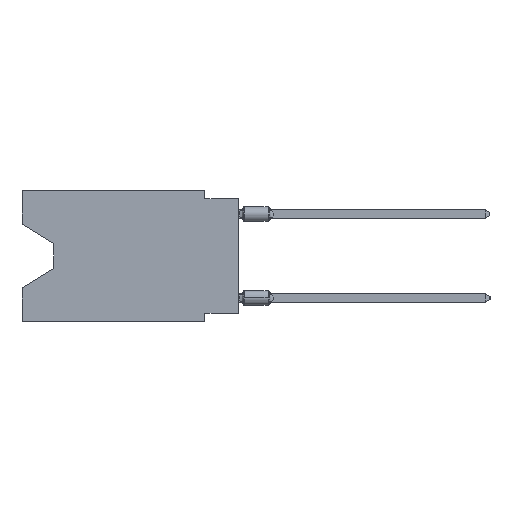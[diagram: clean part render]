
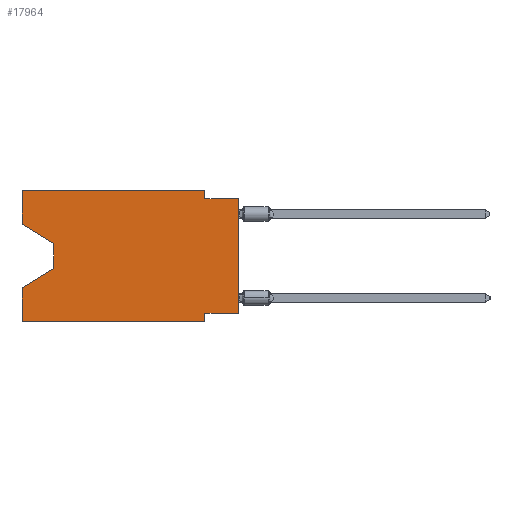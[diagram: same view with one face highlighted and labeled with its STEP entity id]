
A CAD part, left-side view. The second image highlights one B-rep face of the part: STEP entity #17964.
In plain terms, the highlighted planar face has unit normal (-1, 0, 0).
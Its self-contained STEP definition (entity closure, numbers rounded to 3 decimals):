
#2593 = LINE ( 'NONE', #3470, #9053 ) ;
#2955 = VERTEX_POINT ( 'NONE', #20344 ) ;
#3470 = CARTESIAN_POINT ( 'NONE',  ( 0., 0., -0.635 ) ) ;
#4074 = CARTESIAN_POINT ( 'NONE',  ( 0., 16.383, -2.546 ) ) ;
#4353 = LINE ( 'NONE', #4074, #47455 ) ;
#4602 = DIRECTION ( 'NONE',  ( 0., 1., 0. ) ) ;
#5202 = ORIENTED_EDGE ( 'NONE', *, *, #27880, .T. ) ;
#5480 = EDGE_CURVE ( 'NONE', #35340, #27642, #8712, .T. ) ;
#5612 = PLANE ( 'NONE',  #28601 ) ;
#5789 = DIRECTION ( 'NONE',  ( 0., -1., 0. ) ) ;
#5990 = ORIENTED_EDGE ( 'NONE', *, *, #41728, .F. ) ;
#7350 = EDGE_CURVE ( 'NONE', #36965, #53989, #55709, .T. ) ;
#8078 = VERTEX_POINT ( 'NONE', #9866 ) ;
#8114 = CARTESIAN_POINT ( 'NONE',  ( 0., 0., -9.271 ) ) ;
#8610 = EDGE_CURVE ( 'NONE', #47030, #40802, #19693, .T. ) ;
#8712 = LINE ( 'NONE', #17474, #56254 ) ;
#9053 = VECTOR ( 'NONE', #56425, 1000. ) ;
#9615 = VERTEX_POINT ( 'NONE', #36421 ) ;
#9800 = CARTESIAN_POINT ( 'NONE',  ( 0., 13.97, -4.013 ) ) ;
#9866 = CARTESIAN_POINT ( 'NONE',  ( 0., 13.97, -5.893 ) ) ;
#10075 = LINE ( 'NONE', #9800, #38184 ) ;
#10081 = CARTESIAN_POINT ( 'NONE',  ( 0., 2.54, 0. ) ) ;
#10205 = EDGE_CURVE ( 'NONE', #35075, #56431, #42723, .T. ) ;
#10977 = CARTESIAN_POINT ( 'NONE',  ( 0., 16.383, -2.546 ) ) ;
#11477 = CARTESIAN_POINT ( 'NONE',  ( 0., 16.383, -9.906 ) ) ;
#11584 = ORIENTED_EDGE ( 'NONE', *, *, #8610, .T. ) ;
#12892 = DIRECTION ( 'NONE',  ( 0., 0., 1. ) ) ;
#13068 = CARTESIAN_POINT ( 'NONE',  ( 0., 0., -0.635 ) ) ;
#13733 = VECTOR ( 'NONE', #12892, 1000. ) ;
#15483 = VECTOR ( 'NONE', #55414, 1000. ) ;
#16122 = CARTESIAN_POINT ( 'NONE',  ( 0., 16.383, 0. ) ) ;
#17239 = DIRECTION ( 'NONE',  ( 0., 0.855, -0.519 ) ) ;
#17474 = CARTESIAN_POINT ( 'NONE',  ( 0., 16.383, 0. ) ) ;
#17768 = DIRECTION ( 'NONE',  ( 0., 0., 1. ) ) ;
#17964 = ADVANCED_FACE ( 'NONE', ( #55345 ), #5612, .F. ) ;
#18504 = EDGE_CURVE ( 'NONE', #53989, #40802, #2593, .T. ) ;
#19154 = ORIENTED_EDGE ( 'NONE', *, *, #18504, .F. ) ;
#19693 = LINE ( 'NONE', #37544, #15483 ) ;
#20344 = CARTESIAN_POINT ( 'NONE',  ( 0., 13.97, -4.013 ) ) ;
#20824 = VECTOR ( 'NONE', #21401, 1000. ) ;
#21401 = DIRECTION ( 'NONE',  ( 0., -1., 0. ) ) ;
#22155 = EDGE_CURVE ( 'NONE', #47030, #34508, #52581, .T. ) ;
#23251 = ORIENTED_EDGE ( 'NONE', *, *, #31248, .T. ) ;
#23791 = DIRECTION ( 'NONE',  ( 0., 0., -1. ) ) ;
#25501 = LINE ( 'NONE', #11477, #20824 ) ;
#25913 = ORIENTED_EDGE ( 'NONE', *, *, #36731, .T. ) ;
#27325 = CARTESIAN_POINT ( 'NONE',  ( 0., 16.383, -9.906 ) ) ;
#27642 = VERTEX_POINT ( 'NONE', #51492 ) ;
#27869 = EDGE_LOOP ( 'NONE', ( #27938, #23251, #5202, #39796, #25913, #41857, #35771, #11584, #19154, #55589, #5990, #55745 ) ) ;
#27880 = EDGE_CURVE ( 'NONE', #8078, #27642, #35365, .T. ) ;
#27938 = ORIENTED_EDGE ( 'NONE', *, *, #45443, .T. ) ;
#28122 = DIRECTION ( 'NONE',  ( 1., 0., 0. ) ) ;
#28601 = AXIS2_PLACEMENT_3D ( 'NONE', #32797, #28122, #55628 ) ;
#30107 = VECTOR ( 'NONE', #55307, 1000. ) ;
#31248 = EDGE_CURVE ( 'NONE', #2955, #8078, #10075, .T. ) ;
#31757 = VECTOR ( 'NONE', #4602, 1000. ) ;
#32797 = CARTESIAN_POINT ( 'NONE',  ( 0., 16.383, 0. ) ) ;
#34508 = VERTEX_POINT ( 'NONE', #41472 ) ;
#35075 = VERTEX_POINT ( 'NONE', #10977 ) ;
#35340 = VERTEX_POINT ( 'NONE', #27325 ) ;
#35365 = LINE ( 'NONE', #53223, #54873 ) ;
#35771 = ORIENTED_EDGE ( 'NONE', *, *, #22155, .F. ) ;
#36421 = CARTESIAN_POINT ( 'NONE',  ( 0., 2.54, -9.906 ) ) ;
#36731 = EDGE_CURVE ( 'NONE', #35340, #9615, #25501, .T. ) ;
#36965 = VERTEX_POINT ( 'NONE', #45381 ) ;
#37544 = CARTESIAN_POINT ( 'NONE',  ( 0., 0., 0. ) ) ;
#37719 = CARTESIAN_POINT ( 'NONE',  ( 0., 2.54, -9.906 ) ) ;
#37820 = VECTOR ( 'NONE', #5789, 1000. ) ;
#38184 = VECTOR ( 'NONE', #41077, 1000. ) ;
#39220 = CARTESIAN_POINT ( 'NONE',  ( 0., 16.383, 0. ) ) ;
#39796 = ORIENTED_EDGE ( 'NONE', *, *, #5480, .F. ) ;
#40802 = VERTEX_POINT ( 'NONE', #13068 ) ;
#41077 = DIRECTION ( 'NONE',  ( 0., 0., -1. ) ) ;
#41472 = CARTESIAN_POINT ( 'NONE',  ( 0., 2.54, -9.271 ) ) ;
#41728 = EDGE_CURVE ( 'NONE', #56431, #36965, #41747, .T. ) ;
#41747 = LINE ( 'NONE', #47010, #37820 ) ;
#41857 = ORIENTED_EDGE ( 'NONE', *, *, #50854, .F. ) ;
#42723 = LINE ( 'NONE', #39220, #13733 ) ;
#44426 = DIRECTION ( 'NONE',  ( 0., -0.855, -0.519 ) ) ;
#45381 = CARTESIAN_POINT ( 'NONE',  ( 0., 2.54, 0. ) ) ;
#45443 = EDGE_CURVE ( 'NONE', #35075, #2955, #4353, .T. ) ;
#47010 = CARTESIAN_POINT ( 'NONE',  ( 0., 16.383, 0. ) ) ;
#47030 = VERTEX_POINT ( 'NONE', #55527 ) ;
#47455 = VECTOR ( 'NONE', #44426, 1000. ) ;
#48078 = VECTOR ( 'NONE', #23791, 1000. ) ;
#50854 = EDGE_CURVE ( 'NONE', #34508, #9615, #50902, .T. ) ;
#50902 = LINE ( 'NONE', #37719, #30107 ) ;
#51123 = CARTESIAN_POINT ( 'NONE',  ( 0., 2.54, -0.635 ) ) ;
#51492 = CARTESIAN_POINT ( 'NONE',  ( 0., 16.383, -7.36 ) ) ;
#52581 = LINE ( 'NONE', #8114, #31757 ) ;
#53223 = CARTESIAN_POINT ( 'NONE',  ( 0., 13.97, -5.893 ) ) ;
#53989 = VERTEX_POINT ( 'NONE', #51123 ) ;
#54873 = VECTOR ( 'NONE', #17239, 1000. ) ;
#55307 = DIRECTION ( 'NONE',  ( 0., 0., -1. ) ) ;
#55345 = FACE_OUTER_BOUND ( 'NONE', #27869, .T. ) ;
#55414 = DIRECTION ( 'NONE',  ( 0., 0., 1. ) ) ;
#55527 = CARTESIAN_POINT ( 'NONE',  ( 0., 0., -9.271 ) ) ;
#55589 = ORIENTED_EDGE ( 'NONE', *, *, #7350, .F. ) ;
#55628 = DIRECTION ( 'NONE',  ( 0., 0., -1. ) ) ;
#55709 = LINE ( 'NONE', #10081, #48078 ) ;
#55745 = ORIENTED_EDGE ( 'NONE', *, *, #10205, .F. ) ;
#56254 = VECTOR ( 'NONE', #17768, 1000. ) ;
#56425 = DIRECTION ( 'NONE',  ( 0., -1., 0. ) ) ;
#56431 = VERTEX_POINT ( 'NONE', #16122 ) ;
